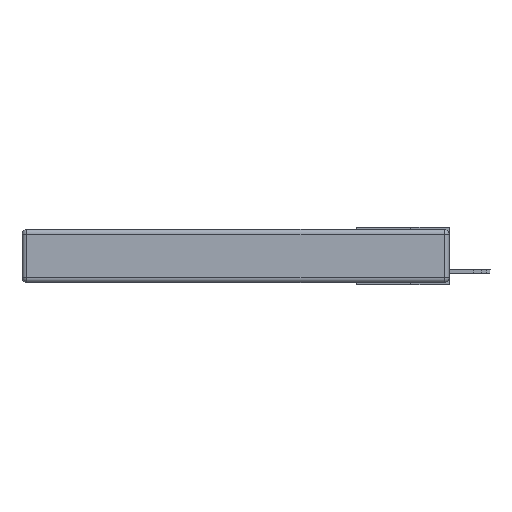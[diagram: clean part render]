
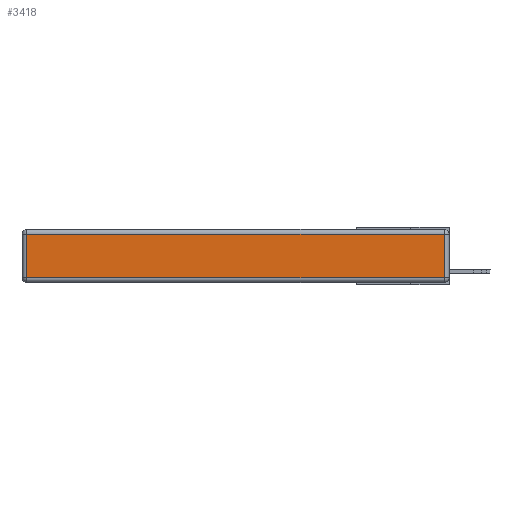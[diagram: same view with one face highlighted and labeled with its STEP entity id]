
A CAD part, left-side view. The second image highlights one B-rep face of the part: STEP entity #3418.
In plain terms, the highlighted planar face has unit normal (-1, 0, 0).
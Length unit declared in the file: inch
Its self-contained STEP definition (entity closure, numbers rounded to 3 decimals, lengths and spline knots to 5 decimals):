
#1500 = EDGE_CURVE ( 'NONE', #6883, #10079, #10770, .T. ) ;
#2201 = DIRECTION ( 'NONE',  ( 0., 1., 0. ) ) ;
#2310 = EDGE_LOOP ( 'NONE', ( #7284, #7479, #5759, #8356 ) ) ;
#2850 = LINE ( 'NONE', #10215, #5057 ) ;
#3045 = VECTOR ( 'NONE', #6189, 39.37008 ) ;
#3411 = VERTEX_POINT ( 'NONE', #8100 ) ;
#3418 = ADVANCED_FACE ( 'NONE', ( #9474 ), #10057, .T. ) ;
#4732 = CARTESIAN_POINT ( 'NONE',  ( 0., 0.03, -0.313 ) ) ;
#5057 = VECTOR ( 'NONE', #2201, 39.37008 ) ;
#5361 = DIRECTION ( 'NONE',  ( 0., 0., 1. ) ) ;
#5759 = ORIENTED_EDGE ( 'NONE', *, *, #10151, .T. ) ;
#5970 = CARTESIAN_POINT ( 'NONE',  ( 0., 2.72, -0.313 ) ) ;
#6189 = DIRECTION ( 'NONE',  ( 0., 0., -1. ) ) ;
#6347 = LINE ( 'NONE', #12281, #3045 ) ;
#6883 = VERTEX_POINT ( 'NONE', #5970 ) ;
#7074 = DIRECTION ( 'NONE',  ( -1., 0., 0. ) ) ;
#7284 = ORIENTED_EDGE ( 'NONE', *, *, #1500, .T. ) ;
#7479 = ORIENTED_EDGE ( 'NONE', *, *, #12896, .T. ) ;
#7482 = VERTEX_POINT ( 'NONE', #9461 ) ;
#8100 = CARTESIAN_POINT ( 'NONE',  ( 0., 0.03, -0.03 ) ) ;
#8356 = ORIENTED_EDGE ( 'NONE', *, *, #8626, .T. ) ;
#8574 = CARTESIAN_POINT ( 'NONE',  ( 0., 0., -0.313 ) ) ;
#8626 = EDGE_CURVE ( 'NONE', #7482, #6883, #6347, .T. ) ;
#9412 = VECTOR ( 'NONE', #5361, 39.37008 ) ;
#9461 = CARTESIAN_POINT ( 'NONE',  ( 0., 2.72, -0.03 ) ) ;
#9474 = FACE_OUTER_BOUND ( 'NONE', #2310, .T. ) ;
#10057 = PLANE ( 'NONE',  #12007 ) ;
#10079 = VERTEX_POINT ( 'NONE', #4732 ) ;
#10151 = EDGE_CURVE ( 'NONE', #3411, #7482, #2850, .T. ) ;
#10215 = CARTESIAN_POINT ( 'NONE',  ( 0., 2.75, -0.03 ) ) ;
#10624 = VECTOR ( 'NONE', #12696, 39.37008 ) ;
#10770 = LINE ( 'NONE', #8574, #10624 ) ;
#11076 = CARTESIAN_POINT ( 'NONE',  ( 0., 0., -0.343 ) ) ;
#11473 = CARTESIAN_POINT ( 'NONE',  ( 0., 0.03, -0.343 ) ) ;
#12007 = AXIS2_PLACEMENT_3D ( 'NONE', #11076, #7074, #12103 ) ;
#12103 = DIRECTION ( 'NONE',  ( 0., 0., 1. ) ) ;
#12281 = CARTESIAN_POINT ( 'NONE',  ( 0., 2.72, -0.343 ) ) ;
#12696 = DIRECTION ( 'NONE',  ( 0., -1., 0. ) ) ;
#12862 = LINE ( 'NONE', #11473, #9412 ) ;
#12896 = EDGE_CURVE ( 'NONE', #10079, #3411, #12862, .T. ) ;
